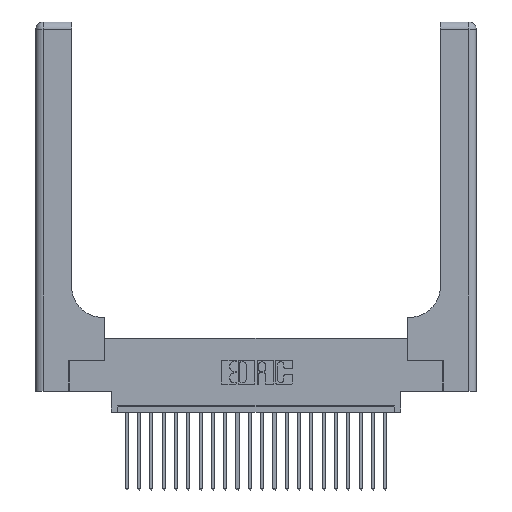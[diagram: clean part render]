
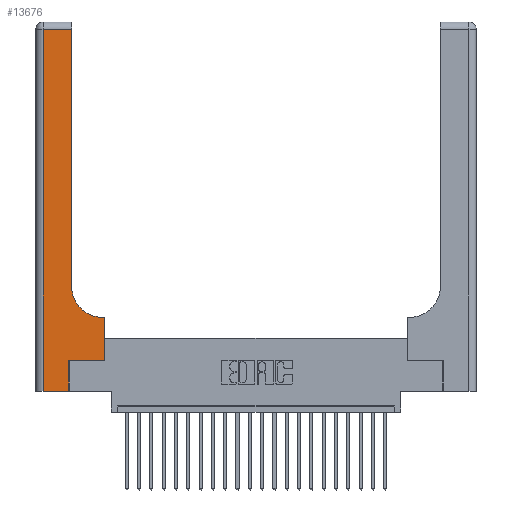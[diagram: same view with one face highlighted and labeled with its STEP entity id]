
A CAD part, top view. The second image highlights one B-rep face of the part: STEP entity #13676.
In plain terms, the highlighted planar face has unit normal (0, 0, 1).
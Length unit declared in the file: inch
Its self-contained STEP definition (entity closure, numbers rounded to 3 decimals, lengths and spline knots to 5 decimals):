
#633 = CARTESIAN_POINT ( 'NONE',  ( 0.5585, 0.25, 0.37 ) ) ;
#869 = CARTESIAN_POINT ( 'NONE',  ( 0.5415, 0.85, 0.37 ) ) ;
#1508 = CARTESIAN_POINT ( 'NONE',  ( 0., 2.94, 0.37 ) ) ;
#2003 = EDGE_CURVE ( 'NONE', #15499, #8410, #13878, .T. ) ;
#2380 = DIRECTION ( 'NONE',  ( 1., 0., 0. ) ) ;
#3330 = LINE ( 'NONE', #12198, #6639 ) ;
#3616 = EDGE_CURVE ( 'NONE', #4048, #15499, #22360, .T. ) ;
#3787 = CARTESIAN_POINT ( 'NONE',  ( 0.269, 0.25, 0.37 ) ) ;
#3986 = DIRECTION ( 'NONE',  ( 0., 1., 0. ) ) ;
#4012 = ORIENTED_EDGE ( 'NONE', *, *, #5990, .T. ) ;
#4048 = VERTEX_POINT ( 'NONE', #11635 ) ;
#4090 = CARTESIAN_POINT ( 'NONE',  ( 0.2915, 0.6, 0.37 ) ) ;
#4145 = LINE ( 'NONE', #24609, #23360 ) ;
#4167 = DIRECTION ( 'NONE',  ( -1., 0., 0. ) ) ;
#5125 = VECTOR ( 'NONE', #4167, 39.37008 ) ;
#5384 = EDGE_CURVE ( 'NONE', #8453, #11390, #9873, .T. ) ;
#5435 = VECTOR ( 'NONE', #19130, 39.37008 ) ;
#5589 = VECTOR ( 'NONE', #9075, 39.37008 ) ;
#5808 = ORIENTED_EDGE ( 'NONE', *, *, #11520, .T. ) ;
#5990 = EDGE_CURVE ( 'NONE', #19318, #11156, #21647, .T. ) ;
#6639 = VECTOR ( 'NONE', #15728, 39.37008 ) ;
#6792 = ORIENTED_EDGE ( 'NONE', *, *, #2003, .T. ) ;
#7911 = ORIENTED_EDGE ( 'NONE', *, *, #11552, .T. ) ;
#8410 = VERTEX_POINT ( 'NONE', #24268 ) ;
#8453 = VERTEX_POINT ( 'NONE', #22117 ) ;
#8547 = ORIENTED_EDGE ( 'NONE', *, *, #14315, .T. ) ;
#9075 = DIRECTION ( 'NONE',  ( -1., 0., 0. ) ) ;
#9253 = LINE ( 'NONE', #4090, #5125 ) ;
#9873 = LINE ( 'NONE', #13765, #19348 ) ;
#10172 = ORIENTED_EDGE ( 'NONE', *, *, #3616, .T. ) ;
#10627 = CARTESIAN_POINT ( 'NONE',  ( 0.2915, 0.85, 0.37 ) ) ;
#11156 = VERTEX_POINT ( 'NONE', #633 ) ;
#11390 = VERTEX_POINT ( 'NONE', #18808 ) ;
#11520 = EDGE_CURVE ( 'NONE', #15581, #8453, #11665, .T. ) ;
#11552 = EDGE_CURVE ( 'NONE', #11390, #19318, #3330, .T. ) ;
#11635 = CARTESIAN_POINT ( 'NONE',  ( 0.5415, 0.6, 0.37 ) ) ;
#11665 = LINE ( 'NONE', #11879, #5435 ) ;
#11879 = CARTESIAN_POINT ( 'NONE',  ( 0.06, 3., 0.37 ) ) ;
#12081 = VECTOR ( 'NONE', #15996, 39.37008 ) ;
#12198 = CARTESIAN_POINT ( 'NONE',  ( 0.269, 0., 0.37 ) ) ;
#12207 = CARTESIAN_POINT ( 'NONE',  ( 0.5585, 0.6, 0.37 ) ) ;
#13437 = VERTEX_POINT ( 'NONE', #12207 ) ;
#13676 = ADVANCED_FACE ( 'NONE', ( #20192 ), #18298, .F. ) ;
#13765 = CARTESIAN_POINT ( 'NONE',  ( 0., 0., 0.37 ) ) ;
#13878 = LINE ( 'NONE', #22451, #12081 ) ;
#13920 = AXIS2_PLACEMENT_3D ( 'NONE', #20500, #16624, #24372 ) ;
#14315 = EDGE_CURVE ( 'NONE', #11156, #13437, #4145, .T. ) ;
#14484 = ORIENTED_EDGE ( 'NONE', *, *, #5384, .T. ) ;
#15499 = VERTEX_POINT ( 'NONE', #10627 ) ;
#15581 = VERTEX_POINT ( 'NONE', #23844 ) ;
#15652 = AXIS2_PLACEMENT_3D ( 'NONE', #869, #19806, #19630 ) ;
#15728 = DIRECTION ( 'NONE',  ( 0., 1., 0. ) ) ;
#15996 = DIRECTION ( 'NONE',  ( 0., 1., 0. ) ) ;
#16624 = DIRECTION ( 'NONE',  ( 0., 0., -1. ) ) ;
#16737 = ORIENTED_EDGE ( 'NONE', *, *, #17541, .T. ) ;
#16865 = LINE ( 'NONE', #1508, #5589 ) ;
#17361 = CARTESIAN_POINT ( 'NONE',  ( 0.269, 0.25, 0.37 ) ) ;
#17541 = EDGE_CURVE ( 'NONE', #13437, #4048, #9253, .T. ) ;
#18128 = VECTOR ( 'NONE', #21135, 39.37008 ) ;
#18298 = PLANE ( 'NONE',  #13920 ) ;
#18338 = EDGE_LOOP ( 'NONE', ( #6792, #22962, #5808, #14484, #7911, #4012, #8547, #16737, #10172 ) ) ;
#18808 = CARTESIAN_POINT ( 'NONE',  ( 0.269, 0., 0.37 ) ) ;
#19130 = DIRECTION ( 'NONE',  ( 0., -1., 0. ) ) ;
#19318 = VERTEX_POINT ( 'NONE', #3787 ) ;
#19348 = VECTOR ( 'NONE', #2380, 39.37008 ) ;
#19630 = DIRECTION ( 'NONE',  ( 1., 0., 0. ) ) ;
#19640 = EDGE_CURVE ( 'NONE', #8410, #15581, #16865, .T. ) ;
#19806 = DIRECTION ( 'NONE',  ( 0., 0., -1. ) ) ;
#20192 = FACE_OUTER_BOUND ( 'NONE', #18338, .T. ) ;
#20500 = CARTESIAN_POINT ( 'NONE',  ( 0., 3., 0.37 ) ) ;
#21135 = DIRECTION ( 'NONE',  ( 1., 0., 0. ) ) ;
#21647 = LINE ( 'NONE', #17361, #18128 ) ;
#22117 = CARTESIAN_POINT ( 'NONE',  ( 0.06, 0., 0.37 ) ) ;
#22360 = CIRCLE ( 'NONE', #15652, 0.25 ) ;
#22451 = CARTESIAN_POINT ( 'NONE',  ( 0.2915, 3., 0.37 ) ) ;
#22962 = ORIENTED_EDGE ( 'NONE', *, *, #19640, .T. ) ;
#23360 = VECTOR ( 'NONE', #3986, 39.37008 ) ;
#23844 = CARTESIAN_POINT ( 'NONE',  ( 0.06, 2.94, 0.37 ) ) ;
#24268 = CARTESIAN_POINT ( 'NONE',  ( 0.2915, 2.94, 0.37 ) ) ;
#24372 = DIRECTION ( 'NONE',  ( -1., 0., 0. ) ) ;
#24609 = CARTESIAN_POINT ( 'NONE',  ( 0.5585, 0.25, 0.37 ) ) ;
